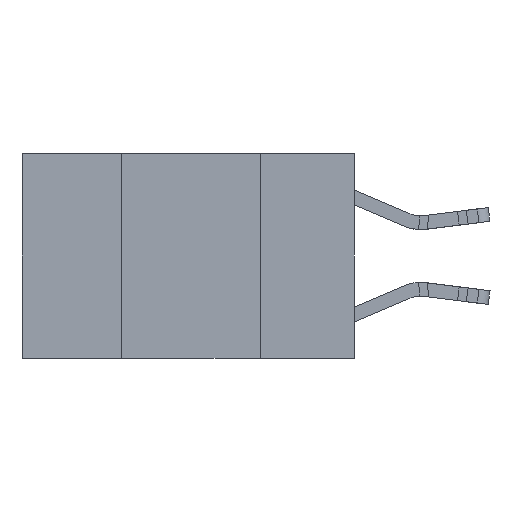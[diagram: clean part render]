
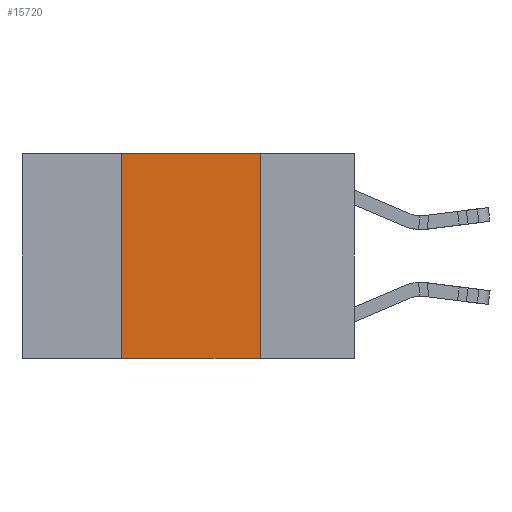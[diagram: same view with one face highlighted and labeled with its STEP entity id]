
A CAD part, left-side view. The second image highlights one B-rep face of the part: STEP entity #15720.
In plain terms, the highlighted planar face has unit normal (-1, 0, 0).
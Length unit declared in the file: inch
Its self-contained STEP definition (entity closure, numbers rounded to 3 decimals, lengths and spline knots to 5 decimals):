
#757 = VECTOR ( 'NONE', #13088, 39.37008 ) ;
#1109 = CARTESIAN_POINT ( 'NONE',  ( 0., 0.42, -0.37 ) ) ;
#1552 = CARTESIAN_POINT ( 'NONE',  ( 0., 0.17, 0. ) ) ;
#3088 = LINE ( 'NONE', #9842, #14555 ) ;
#3870 = CARTESIAN_POINT ( 'NONE',  ( 0., 0.6, 0. ) ) ;
#4868 = VERTEX_POINT ( 'NONE', #6823 ) ;
#5927 = CARTESIAN_POINT ( 'NONE',  ( 0., 0.42, 0. ) ) ;
#6823 = CARTESIAN_POINT ( 'NONE',  ( 0., 0.42, 0. ) ) ;
#7047 = DIRECTION ( 'NONE',  ( 1., 0., 0. ) ) ;
#7584 = ORIENTED_EDGE ( 'NONE', *, *, #21243, .T. ) ;
#8249 = ORIENTED_EDGE ( 'NONE', *, *, #19029, .F. ) ;
#9842 = CARTESIAN_POINT ( 'NONE',  ( 0., 0.17, 0. ) ) ;
#9993 = VERTEX_POINT ( 'NONE', #1552 ) ;
#11020 = CARTESIAN_POINT ( 'NONE',  ( 0., 0.6, -0.37 ) ) ;
#12369 = EDGE_CURVE ( 'NONE', #9993, #15346, #3088, .T. ) ;
#12938 = LINE ( 'NONE', #11020, #18971 ) ;
#13088 = DIRECTION ( 'NONE',  ( 0., -1., 0. ) ) ;
#14555 = VECTOR ( 'NONE', #23419, 39.37008 ) ;
#15346 = VERTEX_POINT ( 'NONE', #23973 ) ;
#15439 = EDGE_CURVE ( 'NONE', #4868, #9993, #25693, .T. ) ;
#15720 = ADVANCED_FACE ( 'NONE', ( #23188 ), #16178, .F. ) ;
#16178 = PLANE ( 'NONE',  #27768 ) ;
#17403 = EDGE_LOOP ( 'NONE', ( #20425, #22508, #8249, #7584 ) ) ;
#17630 = VERTEX_POINT ( 'NONE', #1109 ) ;
#17989 = LINE ( 'NONE', #5927, #29327 ) ;
#18433 = CARTESIAN_POINT ( 'NONE',  ( 0., 0.6, 0. ) ) ;
#18971 = VECTOR ( 'NONE', #29170, 39.37008 ) ;
#19029 = EDGE_CURVE ( 'NONE', #17630, #4868, #17989, .T. ) ;
#20425 = ORIENTED_EDGE ( 'NONE', *, *, #12369, .F. ) ;
#21243 = EDGE_CURVE ( 'NONE', #17630, #15346, #12938, .T. ) ;
#22508 = ORIENTED_EDGE ( 'NONE', *, *, #15439, .F. ) ;
#22987 = DIRECTION ( 'NONE',  ( 0., 0., -1. ) ) ;
#23188 = FACE_OUTER_BOUND ( 'NONE', #17403, .T. ) ;
#23419 = DIRECTION ( 'NONE',  ( 0., 0., -1. ) ) ;
#23973 = CARTESIAN_POINT ( 'NONE',  ( 0., 0.17, -0.37 ) ) ;
#25693 = LINE ( 'NONE', #3870, #757 ) ;
#27768 = AXIS2_PLACEMENT_3D ( 'NONE', #18433, #7047, #22987 ) ;
#28779 = DIRECTION ( 'NONE',  ( 0., 0., 1. ) ) ;
#29170 = DIRECTION ( 'NONE',  ( 0., -1., 0. ) ) ;
#29327 = VECTOR ( 'NONE', #28779, 39.37008 ) ;
